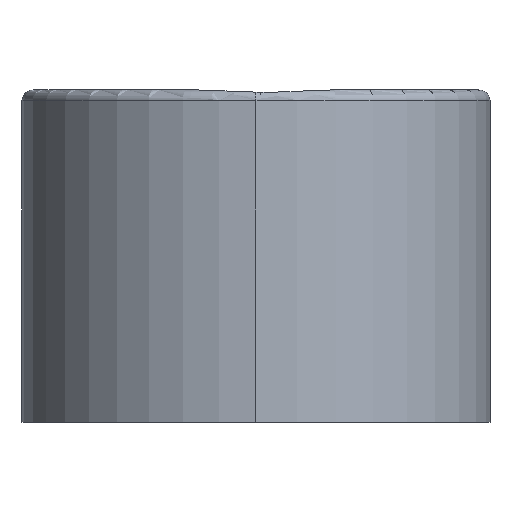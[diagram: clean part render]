
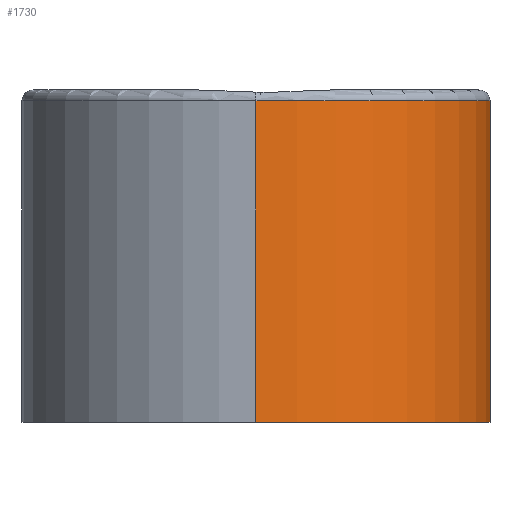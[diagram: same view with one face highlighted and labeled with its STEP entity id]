
A CAD part, front view. The second image highlights one B-rep face of the part: STEP entity #1730.
In plain terms, the highlighted cylindrical face has radius 27 mm (diameter 54 mm), a partial arc.
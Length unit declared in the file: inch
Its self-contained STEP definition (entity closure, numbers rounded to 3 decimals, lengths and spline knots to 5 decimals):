
#73 = EDGE_CURVE ( 'NONE', #1999, #1249, #482, .T. ) ;
#75 = DIRECTION ( 'NONE',  ( 0., 0., -1. ) ) ;
#295 = CARTESIAN_POINT ( 'NONE',  ( 0.10713, -4.74416, 2.99245 ) ) ;
#328 = DIRECTION ( 'NONE',  ( 0., 0., -1. ) ) ;
#343 = AXIS2_PLACEMENT_3D ( 'NONE', #295, #1918, #1926 ) ;
#352 = CARTESIAN_POINT ( 'NONE',  ( 1.17013, -4.74416, 0.44245 ) ) ;
#364 = ORIENTED_EDGE ( 'NONE', *, *, #73, .F. ) ;
#482 = LINE ( 'NONE', #1836, #2881 ) ;
#498 = AXIS2_PLACEMENT_3D ( 'NONE', #1700, #328, #1946 ) ;
#671 = VERTEX_POINT ( 'NONE', #352 ) ;
#684 = CARTESIAN_POINT ( 'NONE',  ( 1.17013, -4.74416, -1.00755 ) ) ;
#837 = ORIENTED_EDGE ( 'NONE', *, *, #1565, .F. ) ;
#865 = DIRECTION ( 'NONE',  ( 0., 0., 1. ) ) ;
#956 = CIRCLE ( 'NONE', #498, 1.06299 ) ;
#1064 = CARTESIAN_POINT ( 'NONE',  ( 0.10713, -4.74416, 0.44245 ) ) ;
#1249 = VERTEX_POINT ( 'NONE', #2029 ) ;
#1259 = VERTEX_POINT ( 'NONE', #684 ) ;
#1297 = EDGE_LOOP ( 'NONE', ( #837, #2688, #364, #2285 ) ) ;
#1308 = DIRECTION ( 'NONE',  ( 0., -1., 0. ) ) ;
#1455 = CARTESIAN_POINT ( 'NONE',  ( 1.17013, -4.74416, -1.00755 ) ) ;
#1465 = VECTOR ( 'NONE', #75, 39.37008 ) ;
#1565 = EDGE_CURVE ( 'NONE', #671, #1259, #2096, .T. ) ;
#1567 = FACE_OUTER_BOUND ( 'NONE', #1297, .T. ) ;
#1663 = AXIS2_PLACEMENT_3D ( 'NONE', #1064, #2706, #1308 ) ;
#1700 = CARTESIAN_POINT ( 'NONE',  ( 0.10713, -4.74416, -1.00755 ) ) ;
#1730 = ADVANCED_FACE ( 'NONE', ( #1567 ), #2753, .T. ) ;
#1762 = EDGE_CURVE ( 'NONE', #1259, #1999, #956, .T. ) ;
#1836 = CARTESIAN_POINT ( 'NONE',  ( 0.11385, -5.80713, 0.99245 ) ) ;
#1918 = DIRECTION ( 'NONE',  ( 0., 0., -1. ) ) ;
#1926 = DIRECTION ( 'NONE',  ( 0., 1., 0. ) ) ;
#1946 = DIRECTION ( 'NONE',  ( 0., 1., 0. ) ) ;
#1999 = VERTEX_POINT ( 'NONE', #2070 ) ;
#2029 = CARTESIAN_POINT ( 'NONE',  ( 0.11385, -5.80713, 0.44245 ) ) ;
#2070 = CARTESIAN_POINT ( 'NONE',  ( 0.11385, -5.80713, -1.00755 ) ) ;
#2080 = EDGE_CURVE ( 'NONE', #671, #1249, #2567, .T. ) ;
#2096 = LINE ( 'NONE', #1455, #1465 ) ;
#2285 = ORIENTED_EDGE ( 'NONE', *, *, #1762, .F. ) ;
#2567 = CIRCLE ( 'NONE', #1663, 1.06299 ) ;
#2688 = ORIENTED_EDGE ( 'NONE', *, *, #2080, .T. ) ;
#2706 = DIRECTION ( 'NONE',  ( 0., 0., -1. ) ) ;
#2753 = CYLINDRICAL_SURFACE ( 'NONE', #343, 1.06299 ) ;
#2881 = VECTOR ( 'NONE', #865, 39.37008 ) ;
